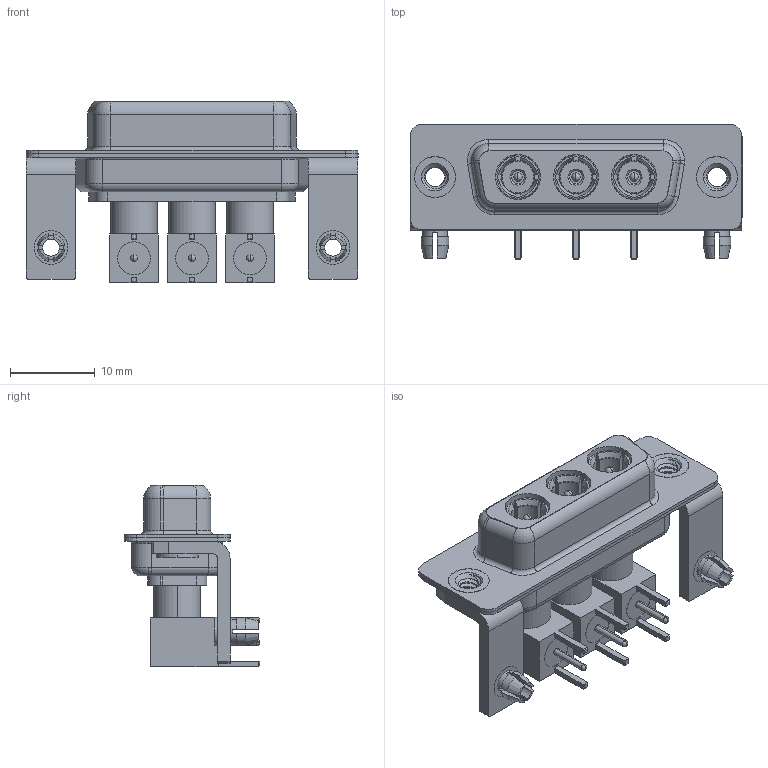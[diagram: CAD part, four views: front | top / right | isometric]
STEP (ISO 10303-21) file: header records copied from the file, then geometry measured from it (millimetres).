
FILE_DESCRIPTION (( 'STEP AP203' ), '1' );
FILE_NAME ('630-3W3-240-7T3.STEP', '2022-05-27T16:50:57', ( '' ), ( '' ), 'SwSTEP 2.0', 'SolidWorks 2020', '' );
FILE_SCHEMA (( 'CONFIG_CONTROL_DESIGN' ));
Length unit declared in the file: millimetre
Products named in the file (16): 630Combo Shell Front_15 Contacts; 630Combo Shell Rear_15 Contacts; Co-Ax Plug Assy_RA; 630Combo Threaded Rivet_3; Co-Ax Plug_RA PC Tail; 630-3W3-240-7T3; Locking Collar; Insulator Pin_Straight PC Tail; 630Combo Board Lock; Pin_RA; 630Combo Housing_3W3; RA Back Shell; 630Combo Stabilizer Bracket; Insulator RA Pin
Assembly tree (30 placements, depth 3):
  630-3W3-240-7T3
    630Combo Housing_3W3
    630Combo Shell Front_15 Contacts
    630Combo Shell Rear_15 Contacts
    630Combo Threaded Rivet_3  x2
    630Combo Stabilizer Bracket  x2
    630Combo Board Lock  x2
    Co-Ax Plug Assy_RA
      Co-Ax Plug_RA PC Tail
      Insulator Pin_Straight PC Tail
      Pin_RA
      Locking Collar
      RA Back Shell
      Insulator RA Pin
    Co-Ax Plug Assy_RA
      Co-Ax Plug_RA PC Tail
      Insulator Pin_Straight PC Tail
      Pin_RA
      Locking Collar
      RA Back Shell
      Insulator RA Pin
    Co-Ax Plug Assy_RA
      Co-Ax Plug_RA PC Tail
      Insulator Pin_Straight PC Tail
      Pin_RA
      Locking Collar
      RA Back Shell
      Insulator RA Pin
Bounding box: 39.2 x 16 x 21.41 mm (x, y, z)
Volume: 3443.4 mm3; surface area: 8586.4 mm2
Topology: 27 solids, 27 shells, 915 faces, 2238 edges, 1410 vertices
Faces by surface type: cylinder 382, plane 336, cone 101, torus 75, sphere 12, bspline 9
Entity records: 18353 total; most frequent: CARTESIAN_POINT 4352, DIRECTION 2680, ORIENTED_EDGE 2384, EDGE_CURVE 1192, AXIS2_PLACEMENT_3D 1071, VERTEX_POINT 755, EDGE_LOOP 553, CIRCLE 549
